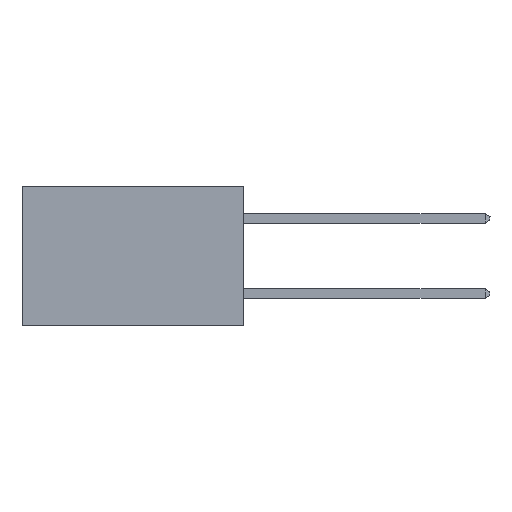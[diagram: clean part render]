
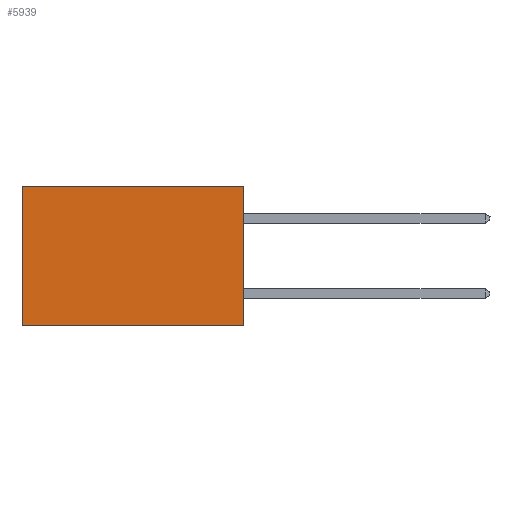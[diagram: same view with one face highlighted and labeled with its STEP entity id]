
A CAD part, left-side view. The second image highlights one B-rep face of the part: STEP entity #5939.
In plain terms, the highlighted planar face has unit normal (-1, 0, 0).
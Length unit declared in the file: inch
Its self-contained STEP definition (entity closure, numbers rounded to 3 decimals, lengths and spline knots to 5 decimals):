
#1135 = VERTEX_POINT ( 'NONE', #13538 ) ;
#1567 = VECTOR ( 'NONE', #10979, 39.37008 ) ;
#1568 = AXIS2_PLACEMENT_3D ( 'NONE', #4833, #11989, #12842 ) ;
#1820 = CARTESIAN_POINT ( 'NONE',  ( 0.277, 0., -0.37 ) ) ;
#2596 = EDGE_CURVE ( 'NONE', #1135, #10607, #11323, .T. ) ;
#3029 = ORIENTED_EDGE ( 'NONE', *, *, #13083, .F. ) ;
#3031 = CARTESIAN_POINT ( 'NONE',  ( 0.277, 0., 0. ) ) ;
#3412 = CARTESIAN_POINT ( 'NONE',  ( 0.277, 0.59, -0.37 ) ) ;
#4746 = CARTESIAN_POINT ( 'NONE',  ( 0.277, 0., -0.37 ) ) ;
#4784 = DIRECTION ( 'NONE',  ( 0., 0., -1. ) ) ;
#4833 = CARTESIAN_POINT ( 'NONE',  ( 0.277, 0., -0.37 ) ) ;
#5469 = ORIENTED_EDGE ( 'NONE', *, *, #13692, .T. ) ;
#5939 = ADVANCED_FACE ( 'NONE', ( #12777 ), #14477, .F. ) ;
#6170 = VERTEX_POINT ( 'NONE', #4746 ) ;
#6306 = DIRECTION ( 'NONE',  ( 0., 1., 0. ) ) ;
#6654 = VERTEX_POINT ( 'NONE', #12376 ) ;
#6919 = LINE ( 'NONE', #7064, #12717 ) ;
#7064 = CARTESIAN_POINT ( 'NONE',  ( 0.277, 0., -0.37 ) ) ;
#7361 = LINE ( 'NONE', #3031, #12788 ) ;
#7796 = VECTOR ( 'NONE', #4784, 39.37008 ) ;
#7993 = EDGE_LOOP ( 'NONE', ( #11073, #3029, #13915, #5469 ) ) ;
#8225 = DIRECTION ( 'NONE',  ( 0., 0., -1. ) ) ;
#8576 = EDGE_CURVE ( 'NONE', #6654, #6170, #6919, .T. ) ;
#10607 = VERTEX_POINT ( 'NONE', #10750 ) ;
#10750 = CARTESIAN_POINT ( 'NONE',  ( 0.277, 0.59, -0.37 ) ) ;
#10979 = DIRECTION ( 'NONE',  ( 0., 1., 0. ) ) ;
#11073 = ORIENTED_EDGE ( 'NONE', *, *, #2596, .T. ) ;
#11323 = LINE ( 'NONE', #3412, #7796 ) ;
#11433 = LINE ( 'NONE', #1820, #1567 ) ;
#11989 = DIRECTION ( 'NONE',  ( 1., 0., 0. ) ) ;
#12376 = CARTESIAN_POINT ( 'NONE',  ( 0.277, 0., 0. ) ) ;
#12717 = VECTOR ( 'NONE', #8225, 39.37008 ) ;
#12777 = FACE_OUTER_BOUND ( 'NONE', #7993, .T. ) ;
#12788 = VECTOR ( 'NONE', #6306, 39.37008 ) ;
#12842 = DIRECTION ( 'NONE',  ( 0., 0., -1. ) ) ;
#13083 = EDGE_CURVE ( 'NONE', #6170, #10607, #11433, .T. ) ;
#13538 = CARTESIAN_POINT ( 'NONE',  ( 0.277, 0.59, 0. ) ) ;
#13692 = EDGE_CURVE ( 'NONE', #6654, #1135, #7361, .T. ) ;
#13915 = ORIENTED_EDGE ( 'NONE', *, *, #8576, .F. ) ;
#14477 = PLANE ( 'NONE',  #1568 ) ;
